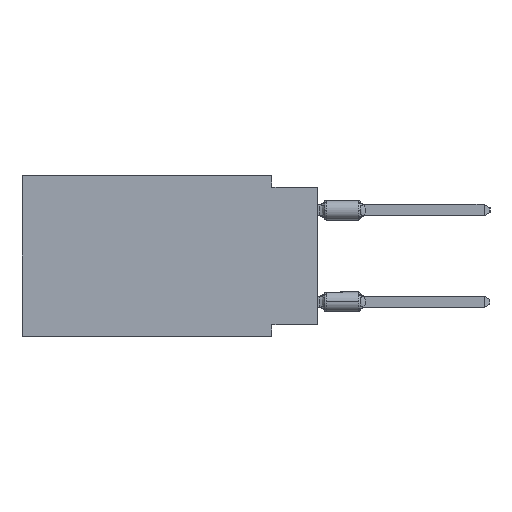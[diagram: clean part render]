
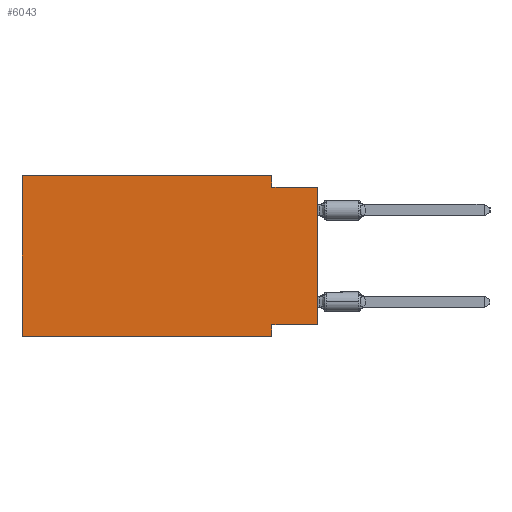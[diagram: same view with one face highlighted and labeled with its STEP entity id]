
A CAD part, left-side view. The second image highlights one B-rep face of the part: STEP entity #6043.
In plain terms, the highlighted planar face has unit normal (-1, 0, 0).
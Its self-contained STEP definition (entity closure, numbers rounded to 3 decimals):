
#370 = VERTEX_POINT ( 'NONE', #12278 ) ;
#1770 = CARTESIAN_POINT ( 'NONE',  ( 0., 0., 0. ) ) ;
#2593 = ORIENTED_EDGE ( 'NONE', *, *, #50552, .F. ) ;
#2723 = EDGE_LOOP ( 'NONE', ( #44643, #11331, #2593, #56567, #53170, #24986, #51855, #21423 ) ) ;
#3776 = VERTEX_POINT ( 'NONE', #52197 ) ;
#4560 = VECTOR ( 'NONE', #34248, 1000. ) ;
#4979 = VECTOR ( 'NONE', #57476, 1000. ) ;
#5238 = VERTEX_POINT ( 'NONE', #11370 ) ;
#6043 = ADVANCED_FACE ( 'NONE', ( #56345 ), #15148, .F. ) ;
#6221 = VERTEX_POINT ( 'NONE', #28674 ) ;
#6862 = LINE ( 'NONE', #1770, #4560 ) ;
#9100 = AXIS2_PLACEMENT_3D ( 'NONE', #33493, #51819, #17730 ) ;
#10176 = DIRECTION ( 'NONE',  ( 0., -1., 0. ) ) ;
#11230 = CARTESIAN_POINT ( 'NONE',  ( 0., 16.383, 0. ) ) ;
#11331 = ORIENTED_EDGE ( 'NONE', *, *, #59007, .F. ) ;
#11370 = CARTESIAN_POINT ( 'NONE',  ( 0., 2.54, -8.89 ) ) ;
#11765 = LINE ( 'NONE', #57466, #30290 ) ;
#11772 = CARTESIAN_POINT ( 'NONE',  ( 0., 0., -0.635 ) ) ;
#12278 = CARTESIAN_POINT ( 'NONE',  ( 0., 16.383, 0. ) ) ;
#12676 = EDGE_CURVE ( 'NONE', #40765, #370, #20228, .T. ) ;
#13573 = DIRECTION ( 'NONE',  ( 0., 0., -1. ) ) ;
#13747 = EDGE_CURVE ( 'NONE', #370, #21602, #21094, .T. ) ;
#15148 = PLANE ( 'NONE',  #9100 ) ;
#16698 = DIRECTION ( 'NONE',  ( 0., 1., 0. ) ) ;
#17166 = CARTESIAN_POINT ( 'NONE',  ( 0., 2.54, 0. ) ) ;
#17730 = DIRECTION ( 'NONE',  ( 0., 0., -1. ) ) ;
#18439 = VERTEX_POINT ( 'NONE', #23779 ) ;
#20228 = LINE ( 'NONE', #11230, #30828 ) ;
#21094 = LINE ( 'NONE', #57793, #46477 ) ;
#21423 = ORIENTED_EDGE ( 'NONE', *, *, #45641, .F. ) ;
#21602 = VERTEX_POINT ( 'NONE', #17166 ) ;
#23779 = CARTESIAN_POINT ( 'NONE',  ( 0., 2.54, -8.255 ) ) ;
#24986 = ORIENTED_EDGE ( 'NONE', *, *, #49626, .T. ) ;
#25726 = LINE ( 'NONE', #44366, #31304 ) ;
#26132 = VECTOR ( 'NONE', #10176, 1000. ) ;
#27571 = CARTESIAN_POINT ( 'NONE',  ( 0., 16.383, -8.89 ) ) ;
#28674 = CARTESIAN_POINT ( 'NONE',  ( 0., 2.54, -0.635 ) ) ;
#30290 = VECTOR ( 'NONE', #31005, 1000. ) ;
#30828 = VECTOR ( 'NONE', #43680, 1000. ) ;
#31005 = DIRECTION ( 'NONE',  ( 0., 0., -1. ) ) ;
#31304 = VECTOR ( 'NONE', #16698, 1000. ) ;
#33025 = LINE ( 'NONE', #51371, #26132 ) ;
#33467 = EDGE_CURVE ( 'NONE', #3776, #52736, #6862, .T. ) ;
#33485 = VECTOR ( 'NONE', #13573, 1000. ) ;
#33493 = CARTESIAN_POINT ( 'NONE',  ( 0., 16.383, 0. ) ) ;
#34248 = DIRECTION ( 'NONE',  ( 0., 0., 1. ) ) ;
#34641 = LINE ( 'NONE', #11772, #4979 ) ;
#35537 = LINE ( 'NONE', #36718, #33485 ) ;
#36130 = DIRECTION ( 'NONE',  ( 0., -1., 0. ) ) ;
#36718 = CARTESIAN_POINT ( 'NONE',  ( 0., 2.54, 0. ) ) ;
#37510 = EDGE_CURVE ( 'NONE', #18439, #5238, #11765, .T. ) ;
#40765 = VERTEX_POINT ( 'NONE', #27571 ) ;
#41394 = CARTESIAN_POINT ( 'NONE',  ( 0., 0., -0.635 ) ) ;
#43680 = DIRECTION ( 'NONE',  ( 0., 0., 1. ) ) ;
#44366 = CARTESIAN_POINT ( 'NONE',  ( 0., 0., -8.255 ) ) ;
#44643 = ORIENTED_EDGE ( 'NONE', *, *, #33467, .T. ) ;
#45641 = EDGE_CURVE ( 'NONE', #3776, #18439, #25726, .T. ) ;
#46477 = VECTOR ( 'NONE', #36130, 1000. ) ;
#49626 = EDGE_CURVE ( 'NONE', #40765, #5238, #33025, .T. ) ;
#50552 = EDGE_CURVE ( 'NONE', #21602, #6221, #35537, .T. ) ;
#51371 = CARTESIAN_POINT ( 'NONE',  ( 0., 16.383, -8.89 ) ) ;
#51819 = DIRECTION ( 'NONE',  ( 1., 0., 0. ) ) ;
#51855 = ORIENTED_EDGE ( 'NONE', *, *, #37510, .F. ) ;
#52197 = CARTESIAN_POINT ( 'NONE',  ( 0., 0., -8.255 ) ) ;
#52736 = VERTEX_POINT ( 'NONE', #41394 ) ;
#53170 = ORIENTED_EDGE ( 'NONE', *, *, #12676, .F. ) ;
#56345 = FACE_OUTER_BOUND ( 'NONE', #2723, .T. ) ;
#56567 = ORIENTED_EDGE ( 'NONE', *, *, #13747, .F. ) ;
#57466 = CARTESIAN_POINT ( 'NONE',  ( 0., 2.54, -8.89 ) ) ;
#57476 = DIRECTION ( 'NONE',  ( 0., -1., 0. ) ) ;
#57793 = CARTESIAN_POINT ( 'NONE',  ( 0., 16.383, 0. ) ) ;
#59007 = EDGE_CURVE ( 'NONE', #6221, #52736, #34641, .T. ) ;
